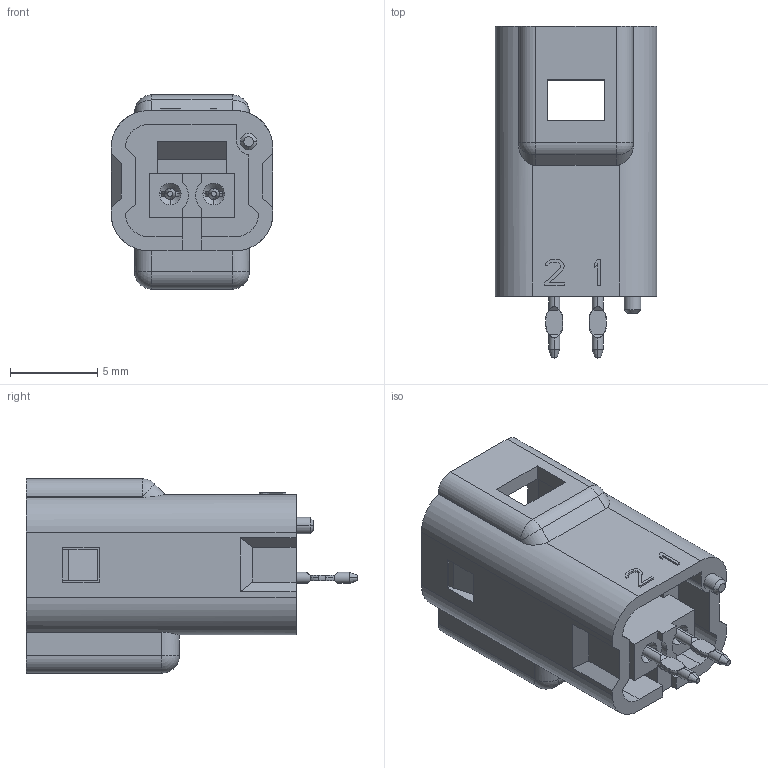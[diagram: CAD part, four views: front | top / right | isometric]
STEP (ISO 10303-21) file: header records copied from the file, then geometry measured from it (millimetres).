
FILE_DESCRIPTION (( 'STEP AP203' ), '1' );
FILE_NAME ('560-002-420-301.STEP', '2020-07-24T16:49:41', ( '' ), ( '' ), 'SwSTEP 2.0', 'SolidWorks 2020', '' );
FILE_SCHEMA (( 'CONFIG_CONTROL_DESIGN' ));
Length unit declared in the file: millimetre
Products named in the file (7): INTERNAL-WIRE-SEAL-2POS; PCB-HEADER-CONTACT-2P; FACIAL-SEAL-2POS; PCB-HEADER-CONTACT-2P-1; 560-002-420-301; PCB-HEADER-HOUSING-2P_BLUE
Assembly tree (6 placements, depth 3):
  560-002-420-301
    560-002-420-301
      PCB-HEADER-HOUSING-2P_BLUE
      PCB-HEADER-CONTACT-2P
      PCB-HEADER-CONTACT-2P-1
      INTERNAL-WIRE-SEAL-2POS
      FACIAL-SEAL-2POS
Bounding box: 9.3 x 19.05 x 11.15 mm (x, y, z)
Volume: 619.9 mm3; surface area: 1816.4 mm2
Topology: 5 solids, 5 shells, 584 faces, 1472 edges, 911 vertices
Faces by surface type: plane 335, cylinder 144, torus 60, cone 41, sphere 4
Entity records: 18250 total; most frequent: CARTESIAN_POINT 3371, DIRECTION 2985, ORIENTED_EDGE 2940, EDGE_CURVE 1470, AXIS2_PLACEMENT_3D 1009, VECTOR 967, LINE 967, VERTEX_POINT 911
